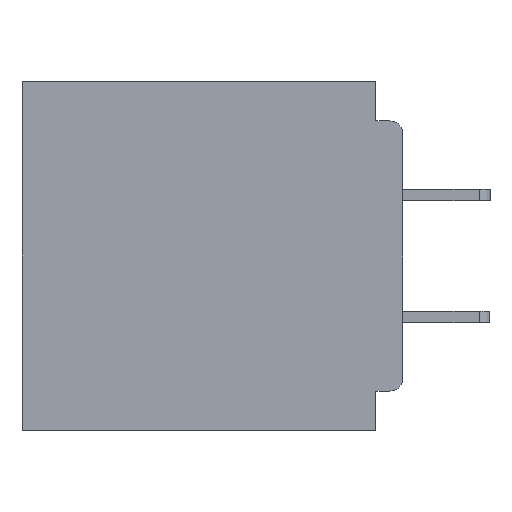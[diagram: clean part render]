
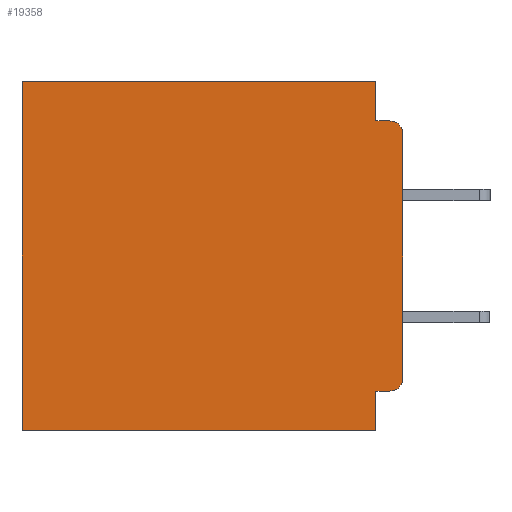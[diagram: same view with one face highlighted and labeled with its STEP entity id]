
A CAD part, left-side view. The second image highlights one B-rep face of the part: STEP entity #19358.
In plain terms, the highlighted planar face has unit normal (-1, 0, 0).
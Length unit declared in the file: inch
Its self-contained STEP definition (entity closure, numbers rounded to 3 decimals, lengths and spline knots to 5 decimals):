
#566 = CARTESIAN_POINT ( 'NONE',  ( 0.3, 0., -0.4 ) ) ;
#923 = DIRECTION ( 'NONE',  ( 0., -1., 0. ) ) ;
#1134 = LINE ( 'NONE', #41388, #29822 ) ;
#1381 = ORIENTED_EDGE ( 'NONE', *, *, #33260, .F. ) ;
#1832 = VECTOR ( 'NONE', #14668, 39.37008 ) ;
#2946 = VERTEX_POINT ( 'NONE', #6108 ) ;
#3394 = DIRECTION ( 'NONE',  ( 0., 0., -1. ) ) ;
#4394 = LINE ( 'NONE', #4675, #23143 ) ;
#4675 = CARTESIAN_POINT ( 'NONE',  ( 0.3, 0., -0.045 ) ) ;
#4908 = VERTEX_POINT ( 'NONE', #19525 ) ;
#5582 = DIRECTION ( 'NONE',  ( 1., 0., 0. ) ) ;
#5795 = CARTESIAN_POINT ( 'NONE',  ( 0.3, 0.031, 0. ) ) ;
#5931 = EDGE_CURVE ( 'NONE', #12029, #41437, #32657, .T. ) ;
#6108 = CARTESIAN_POINT ( 'NONE',  ( 0.3, 0.031, -0.4 ) ) ;
#6747 = VERTEX_POINT ( 'NONE', #38106 ) ;
#7452 = VECTOR ( 'NONE', #34053, 39.37008 ) ;
#7549 = LINE ( 'NONE', #15667, #47301 ) ;
#7868 = VERTEX_POINT ( 'NONE', #26533 ) ;
#8592 = VERTEX_POINT ( 'NONE', #38850 ) ;
#10494 = DIRECTION ( 'NONE',  ( -1., 0., 0. ) ) ;
#10551 = EDGE_LOOP ( 'NONE', ( #1381, #28274, #15999, #24702, #41017, #37511, #25272, #12986, #41479, #24522 ) ) ;
#10766 = VERTEX_POINT ( 'NONE', #32076 ) ;
#11389 = CARTESIAN_POINT ( 'NONE',  ( 0.3, 0.031, -0.045 ) ) ;
#11774 = LINE ( 'NONE', #40579, #1832 ) ;
#12029 = VERTEX_POINT ( 'NONE', #5795 ) ;
#12064 = CARTESIAN_POINT ( 'NONE',  ( 0.3, 0.437, 0. ) ) ;
#12585 = AXIS2_PLACEMENT_3D ( 'NONE', #32882, #10494, #36621 ) ;
#12613 = VECTOR ( 'NONE', #20964, 39.37008 ) ;
#12986 = ORIENTED_EDGE ( 'NONE', *, *, #39587, .F. ) ;
#14668 = DIRECTION ( 'NONE',  ( 0., 0., -1. ) ) ;
#14882 = DIRECTION ( 'NONE',  ( -1., 0., 0. ) ) ;
#15667 = CARTESIAN_POINT ( 'NONE',  ( 0.3, 0., 0. ) ) ;
#15738 = LINE ( 'NONE', #28394, #24488 ) ;
#15999 = ORIENTED_EDGE ( 'NONE', *, *, #34114, .F. ) ;
#16386 = EDGE_CURVE ( 'NONE', #4908, #6747, #1134, .T. ) ;
#17213 = CARTESIAN_POINT ( 'NONE',  ( 0.3, 0., -0.4 ) ) ;
#18315 = CARTESIAN_POINT ( 'NONE',  ( 0.3, 0.031, 0. ) ) ;
#19358 = ADVANCED_FACE ( 'NONE', ( #44752 ), #20475, .F. ) ;
#19525 = CARTESIAN_POINT ( 'NONE',  ( 0.3, 0.015, -0.355 ) ) ;
#20452 = CARTESIAN_POINT ( 'NONE',  ( 0.3, 0., -0.06 ) ) ;
#20475 = PLANE ( 'NONE',  #33683 ) ;
#20964 = DIRECTION ( 'NONE',  ( 0., 0., -1. ) ) ;
#22736 = VECTOR ( 'NONE', #3394, 39.37008 ) ;
#23045 = CIRCLE ( 'NONE', #12585, 0.015 ) ;
#23143 = VECTOR ( 'NONE', #923, 39.37008 ) ;
#24488 = VECTOR ( 'NONE', #32151, 39.37008 ) ;
#24522 = ORIENTED_EDGE ( 'NONE', *, *, #45676, .T. ) ;
#24702 = ORIENTED_EDGE ( 'NONE', *, *, #5931, .F. ) ;
#25272 = ORIENTED_EDGE ( 'NONE', *, *, #40218, .F. ) ;
#26178 = LINE ( 'NONE', #566, #7452 ) ;
#26364 = AXIS2_PLACEMENT_3D ( 'NONE', #37213, #14882, #40958 ) ;
#26533 = CARTESIAN_POINT ( 'NONE',  ( 0.3, 0.015, -0.045 ) ) ;
#28274 = ORIENTED_EDGE ( 'NONE', *, *, #35011, .T. ) ;
#28394 = CARTESIAN_POINT ( 'NONE',  ( 0.3, 0.031, -0.4 ) ) ;
#29822 = VECTOR ( 'NONE', #45170, 39.37008 ) ;
#31586 = CARTESIAN_POINT ( 'NONE',  ( 0.3, 0., -0.4 ) ) ;
#31741 = DIRECTION ( 'NONE',  ( 0., 0., -1. ) ) ;
#32076 = CARTESIAN_POINT ( 'NONE',  ( 0.3, 0.437, -0.4 ) ) ;
#32151 = DIRECTION ( 'NONE',  ( 0., 0., -1. ) ) ;
#32657 = LINE ( 'NONE', #18315, #22736 ) ;
#32882 = CARTESIAN_POINT ( 'NONE',  ( 0.3, 0.015, -0.06 ) ) ;
#33260 = EDGE_CURVE ( 'NONE', #48263, #8592, #42415, .T. ) ;
#33683 = AXIS2_PLACEMENT_3D ( 'NONE', #31586, #5582, #31741 ) ;
#34053 = DIRECTION ( 'NONE',  ( 0., 1., 0. ) ) ;
#34114 = EDGE_CURVE ( 'NONE', #41437, #7868, #4394, .T. ) ;
#35011 = EDGE_CURVE ( 'NONE', #48263, #7868, #23045, .T. ) ;
#36399 = EDGE_CURVE ( 'NONE', #37432, #10766, #11774, .T. ) ;
#36621 = DIRECTION ( 'NONE',  ( 0., 0., -1. ) ) ;
#37213 = CARTESIAN_POINT ( 'NONE',  ( 0.3, 0.015, -0.34 ) ) ;
#37432 = VERTEX_POINT ( 'NONE', #12064 ) ;
#37511 = ORIENTED_EDGE ( 'NONE', *, *, #36399, .T. ) ;
#38106 = CARTESIAN_POINT ( 'NONE',  ( 0.3, 0.031, -0.355 ) ) ;
#38850 = CARTESIAN_POINT ( 'NONE',  ( 0.3, 0., -0.34 ) ) ;
#39308 = EDGE_CURVE ( 'NONE', #12029, #37432, #7549, .T. ) ;
#39587 = EDGE_CURVE ( 'NONE', #6747, #2946, #15738, .T. ) ;
#40194 = CIRCLE ( 'NONE', #26364, 0.015 ) ;
#40218 = EDGE_CURVE ( 'NONE', #2946, #10766, #26178, .T. ) ;
#40579 = CARTESIAN_POINT ( 'NONE',  ( 0.3, 0.437, -0.4 ) ) ;
#40958 = DIRECTION ( 'NONE',  ( 0., 0., -1. ) ) ;
#41017 = ORIENTED_EDGE ( 'NONE', *, *, #39308, .T. ) ;
#41388 = CARTESIAN_POINT ( 'NONE',  ( 0.3, 0., -0.355 ) ) ;
#41437 = VERTEX_POINT ( 'NONE', #11389 ) ;
#41479 = ORIENTED_EDGE ( 'NONE', *, *, #16386, .F. ) ;
#41754 = DIRECTION ( 'NONE',  ( 0., 1., 0. ) ) ;
#42415 = LINE ( 'NONE', #17213, #12613 ) ;
#44752 = FACE_OUTER_BOUND ( 'NONE', #10551, .T. ) ;
#45170 = DIRECTION ( 'NONE',  ( 0., 1., 0. ) ) ;
#45676 = EDGE_CURVE ( 'NONE', #4908, #8592, #40194, .T. ) ;
#47301 = VECTOR ( 'NONE', #41754, 39.37008 ) ;
#48263 = VERTEX_POINT ( 'NONE', #20452 ) ;
